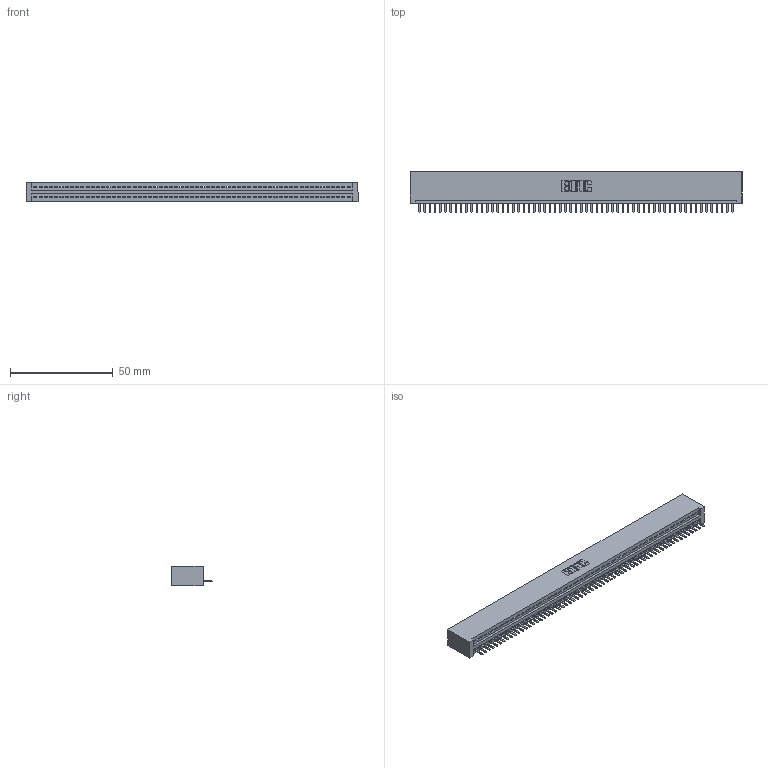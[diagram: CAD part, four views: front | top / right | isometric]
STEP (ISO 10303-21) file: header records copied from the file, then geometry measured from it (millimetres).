
FILE_DESCRIPTION (( 'STEP AP203' ), '1' );
FILE_NAME ('395-061-520-101.STEP', '2019-10-24T13:32:25', ( '' ), ( '' ), 'SwSTEP 2.0', 'SolidWorks 2016', '' );
FILE_SCHEMA (( 'CONFIG_CONTROL_DESIGN' ));
Length unit declared in the file: inch
Products named in the file (3): 395-061-520-101; 345-292-001_345-293-120; 345 Part_No Mounting Lugs
Assembly tree (62 placements, depth 2):
  395-061-520-101
    345 Part_No Mounting Lugs
    345-292-001_345-293-120  x61
Bounding box: 161.54 x 19.68 x 9.4 mm (x, y, z)
Volume: 15908.1 mm3; surface area: 21014.8 mm2
Topology: 62 solids, 62 shells, 3900 faces, 11541 edges, 7530 vertices
Faces by surface type: plane 2638, cylinder 1262
Entity records: 43189 total; most frequent: CARTESIAN_POINT 7499, ORIENTED_EDGE 7482, DIRECTION 6503, EDGE_CURVE 3741, VECTOR 3369, LINE 3369, VERTEX_POINT 2490, AXIS2_PLACEMENT_3D 1567
